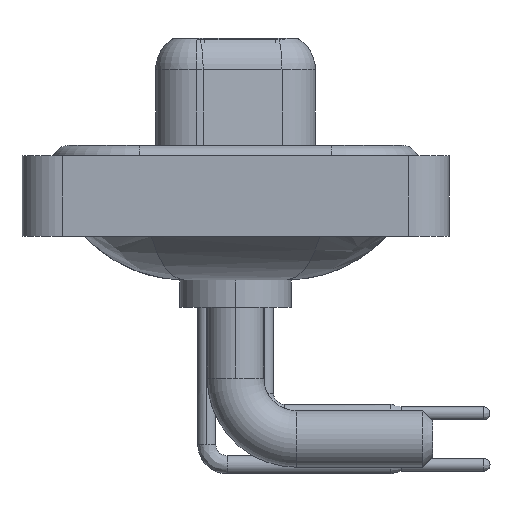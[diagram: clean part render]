
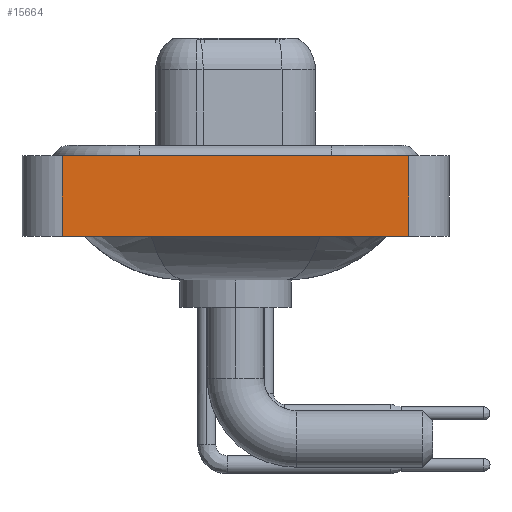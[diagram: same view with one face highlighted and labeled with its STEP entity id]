
A CAD part, left-side view. The second image highlights one B-rep face of the part: STEP entity #15664.
In plain terms, the highlighted planar face has unit normal (-1, 0, 0).
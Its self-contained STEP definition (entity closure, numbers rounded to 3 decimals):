
#780 = ORIENTED_EDGE ( 'NONE', *, *, #14326, .T. ) ;
#1006 = VERTEX_POINT ( 'NONE', #19375 ) ;
#1984 = VECTOR ( 'NONE', #17945, 1000. ) ;
#2395 = CARTESIAN_POINT ( 'NONE',  ( -7.35, -8.55, -3.6 ) ) ;
#2458 = VECTOR ( 'NONE', #2628, 1000. ) ;
#2628 = DIRECTION ( 'NONE',  ( 0., -1., 0. ) ) ;
#3086 = EDGE_LOOP ( 'NONE', ( #3305, #3218, #8003, #780 ) ) ;
#3218 = ORIENTED_EDGE ( 'NONE', *, *, #7390, .F. ) ;
#3305 = ORIENTED_EDGE ( 'NONE', *, *, #11930, .T. ) ;
#4061 = LINE ( 'NONE', #22810, #21551 ) ;
#4126 = FACE_OUTER_BOUND ( 'NONE', #3086, .T. ) ;
#4280 = AXIS2_PLACEMENT_3D ( 'NONE', #21137, #19267, #19144 ) ;
#5480 = DIRECTION ( 'NONE',  ( 0., 0., 1. ) ) ;
#5969 = CARTESIAN_POINT ( 'NONE',  ( -7.35, 8.55, -3.6 ) ) ;
#6090 = LINE ( 'NONE', #2395, #2458 ) ;
#7390 = EDGE_CURVE ( 'NONE', #9713, #9796, #17582, .T. ) ;
#8003 = ORIENTED_EDGE ( 'NONE', *, *, #12906, .F. ) ;
#9713 = VERTEX_POINT ( 'NONE', #14789 ) ;
#9796 = VERTEX_POINT ( 'NONE', #22117 ) ;
#11930 = EDGE_CURVE ( 'NONE', #1006, #9796, #4061, .T. ) ;
#12906 = EDGE_CURVE ( 'NONE', #18949, #9713, #22868, .T. ) ;
#14326 = EDGE_CURVE ( 'NONE', #18949, #1006, #6090, .T. ) ;
#14789 = CARTESIAN_POINT ( 'NONE',  ( -7.35, 8.55, 0.4 ) ) ;
#15235 = DIRECTION ( 'NONE',  ( 0., 0., 1. ) ) ;
#15664 = ADVANCED_FACE ( 'NONE', ( #4126 ), #21023, .T. ) ;
#17582 = LINE ( 'NONE', #23405, #1984 ) ;
#17945 = DIRECTION ( 'NONE',  ( 0., -1., 0. ) ) ;
#18949 = VERTEX_POINT ( 'NONE', #22551 ) ;
#19144 = DIRECTION ( 'NONE',  ( 0., 0., 1. ) ) ;
#19267 = DIRECTION ( 'NONE',  ( -1., 0., 0. ) ) ;
#19375 = CARTESIAN_POINT ( 'NONE',  ( -7.35, -8.55, -3.6 ) ) ;
#20040 = VECTOR ( 'NONE', #5480, 1000. ) ;
#21023 = PLANE ( 'NONE',  #4280 ) ;
#21137 = CARTESIAN_POINT ( 'NONE',  ( -7.35, -8.55, -3.6 ) ) ;
#21551 = VECTOR ( 'NONE', #15235, 1000. ) ;
#22117 = CARTESIAN_POINT ( 'NONE',  ( -7.35, -8.55, 0.4 ) ) ;
#22551 = CARTESIAN_POINT ( 'NONE',  ( -7.35, 8.55, -3.6 ) ) ;
#22810 = CARTESIAN_POINT ( 'NONE',  ( -7.35, -8.55, -3.6 ) ) ;
#22868 = LINE ( 'NONE', #5969, #20040 ) ;
#23405 = CARTESIAN_POINT ( 'NONE',  ( -7.35, -8.55, 0.4 ) ) ;
